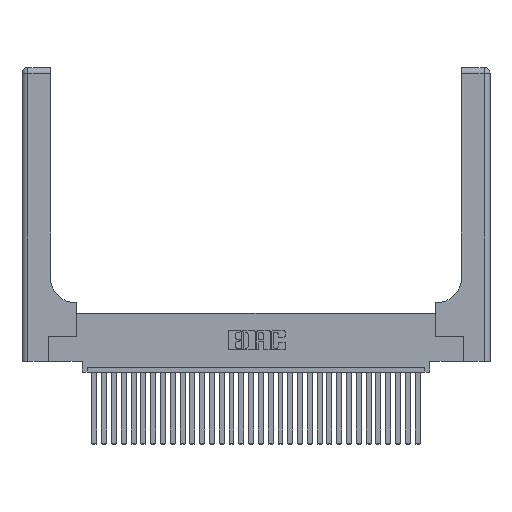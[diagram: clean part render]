
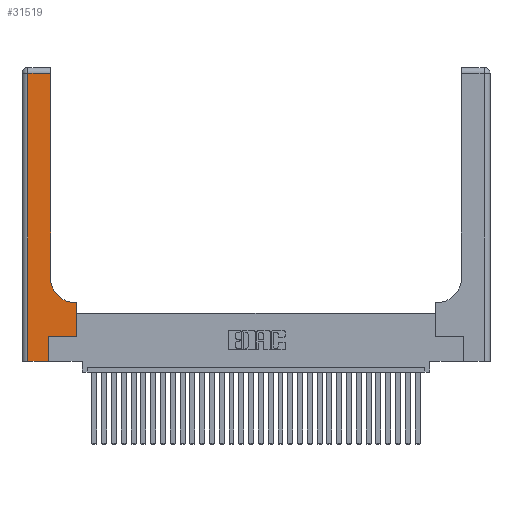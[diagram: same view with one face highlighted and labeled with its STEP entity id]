
A CAD part, top view. The second image highlights one B-rep face of the part: STEP entity #31519.
In plain terms, the highlighted planar face has unit normal (0, 0, 1).
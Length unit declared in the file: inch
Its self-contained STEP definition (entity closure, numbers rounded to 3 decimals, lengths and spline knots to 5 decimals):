
#230 = DIRECTION ( 'NONE',  ( -1., 0., 0. ) ) ;
#403 = CARTESIAN_POINT ( 'NONE',  ( 0.269, 0.25, 0.37 ) ) ;
#1255 = CARTESIAN_POINT ( 'NONE',  ( 0.06, 2.94, 0.37 ) ) ;
#1297 = VERTEX_POINT ( 'NONE', #24731 ) ;
#2402 = ORIENTED_EDGE ( 'NONE', *, *, #20501, .T. ) ;
#2521 = DIRECTION ( 'NONE',  ( 1., 0., 0. ) ) ;
#2644 = VERTEX_POINT ( 'NONE', #13445 ) ;
#3068 = CARTESIAN_POINT ( 'NONE',  ( 0.5585, 0.25, 0.37 ) ) ;
#3902 = ORIENTED_EDGE ( 'NONE', *, *, #19880, .T. ) ;
#4664 = CARTESIAN_POINT ( 'NONE',  ( 0.2915, 3., 0.37 ) ) ;
#4743 = ORIENTED_EDGE ( 'NONE', *, *, #15326, .T. ) ;
#5087 = CARTESIAN_POINT ( 'NONE',  ( 0.5415, 0.85, 0.37 ) ) ;
#5711 = DIRECTION ( 'NONE',  ( 0., 1., 0. ) ) ;
#5930 = FACE_OUTER_BOUND ( 'NONE', #12871, .T. ) ;
#6453 = ORIENTED_EDGE ( 'NONE', *, *, #16240, .T. ) ;
#6502 = CARTESIAN_POINT ( 'NONE',  ( 0., 3., 0.37 ) ) ;
#6890 = EDGE_CURVE ( 'NONE', #15821, #16080, #20571, .T. ) ;
#7287 = CARTESIAN_POINT ( 'NONE',  ( 0.269, 0., 0.37 ) ) ;
#8060 = EDGE_CURVE ( 'NONE', #1297, #13843, #15894, .T. ) ;
#8064 = EDGE_CURVE ( 'NONE', #21628, #1297, #30498, .T. ) ;
#8325 = DIRECTION ( 'NONE',  ( -1., 0., 0. ) ) ;
#8755 = CARTESIAN_POINT ( 'NONE',  ( 0.06, 0., 0.37 ) ) ;
#9092 = CARTESIAN_POINT ( 'NONE',  ( 0., 0., 0.37 ) ) ;
#9494 = LINE ( 'NONE', #11386, #15234 ) ;
#9733 = ORIENTED_EDGE ( 'NONE', *, *, #15636, .T. ) ;
#9889 = CARTESIAN_POINT ( 'NONE',  ( 0.06, 3., 0.37 ) ) ;
#10263 = CARTESIAN_POINT ( 'NONE',  ( 0.269, 0., 0.37 ) ) ;
#10297 = CARTESIAN_POINT ( 'NONE',  ( 0.2915, 2.94, 0.37 ) ) ;
#10461 = AXIS2_PLACEMENT_3D ( 'NONE', #6502, #17881, #8325 ) ;
#10474 = AXIS2_PLACEMENT_3D ( 'NONE', #5087, #22228, #2521 ) ;
#11088 = VERTEX_POINT ( 'NONE', #23471 ) ;
#11386 = CARTESIAN_POINT ( 'NONE',  ( 0., 2.94, 0.37 ) ) ;
#11417 = VERTEX_POINT ( 'NONE', #1255 ) ;
#11964 = VERTEX_POINT ( 'NONE', #10297 ) ;
#12871 = EDGE_LOOP ( 'NONE', ( #9733, #4743, #2402, #18147, #28691, #6453, #15661, #27315, #3902 ) ) ;
#13445 = CARTESIAN_POINT ( 'NONE',  ( 0.2915, 0.85, 0.37 ) ) ;
#13843 = VERTEX_POINT ( 'NONE', #17714 ) ;
#14063 = VECTOR ( 'NONE', #31431, 39.37008 ) ;
#14437 = DIRECTION ( 'NONE',  ( 0., 1., 0. ) ) ;
#14449 = VECTOR ( 'NONE', #14437, 39.37008 ) ;
#14633 = CIRCLE ( 'NONE', #10474, 0.25 ) ;
#15234 = VECTOR ( 'NONE', #230, 39.37008 ) ;
#15326 = EDGE_CURVE ( 'NONE', #11964, #11417, #9494, .T. ) ;
#15636 = EDGE_CURVE ( 'NONE', #2644, #11964, #25500, .T. ) ;
#15661 = ORIENTED_EDGE ( 'NONE', *, *, #8064, .T. ) ;
#15821 = VERTEX_POINT ( 'NONE', #8755 ) ;
#15894 = LINE ( 'NONE', #24783, #31292 ) ;
#16080 = VERTEX_POINT ( 'NONE', #7287 ) ;
#16240 = EDGE_CURVE ( 'NONE', #11088, #21628, #17098, .T. ) ;
#17098 = LINE ( 'NONE', #403, #27413 ) ;
#17714 = CARTESIAN_POINT ( 'NONE',  ( 0.5415, 0.6, 0.37 ) ) ;
#17881 = DIRECTION ( 'NONE',  ( 0., 0., -1. ) ) ;
#18147 = ORIENTED_EDGE ( 'NONE', *, *, #6890, .T. ) ;
#19449 = EDGE_CURVE ( 'NONE', #16080, #11088, #24570, .T. ) ;
#19880 = EDGE_CURVE ( 'NONE', #13843, #2644, #14633, .T. ) ;
#19956 = DIRECTION ( 'NONE',  ( 0., -1., 0. ) ) ;
#20021 = DIRECTION ( 'NONE',  ( 1., 0., 0. ) ) ;
#20225 = DIRECTION ( 'NONE',  ( 0., 1., 0. ) ) ;
#20501 = EDGE_CURVE ( 'NONE', #11417, #15821, #31067, .T. ) ;
#20571 = LINE ( 'NONE', #9092, #14063 ) ;
#21628 = VERTEX_POINT ( 'NONE', #25855 ) ;
#22228 = DIRECTION ( 'NONE',  ( 0., 0., -1. ) ) ;
#23471 = CARTESIAN_POINT ( 'NONE',  ( 0.269, 0.25, 0.37 ) ) ;
#24570 = LINE ( 'NONE', #10263, #31136 ) ;
#24731 = CARTESIAN_POINT ( 'NONE',  ( 0.5585, 0.6, 0.37 ) ) ;
#24783 = CARTESIAN_POINT ( 'NONE',  ( 0.2915, 0.6, 0.37 ) ) ;
#24999 = DIRECTION ( 'NONE',  ( -1., 0., 0. ) ) ;
#25500 = LINE ( 'NONE', #4664, #14449 ) ;
#25855 = CARTESIAN_POINT ( 'NONE',  ( 0.5585, 0.25, 0.37 ) ) ;
#27315 = ORIENTED_EDGE ( 'NONE', *, *, #8060, .T. ) ;
#27413 = VECTOR ( 'NONE', #20021, 39.37008 ) ;
#27951 = VECTOR ( 'NONE', #19956, 39.37008 ) ;
#28691 = ORIENTED_EDGE ( 'NONE', *, *, #19449, .T. ) ;
#30092 = PLANE ( 'NONE',  #10461 ) ;
#30498 = LINE ( 'NONE', #3068, #31659 ) ;
#31067 = LINE ( 'NONE', #9889, #27951 ) ;
#31136 = VECTOR ( 'NONE', #20225, 39.37008 ) ;
#31292 = VECTOR ( 'NONE', #24999, 39.37008 ) ;
#31431 = DIRECTION ( 'NONE',  ( 1., 0., 0. ) ) ;
#31519 = ADVANCED_FACE ( 'NONE', ( #5930 ), #30092, .F. ) ;
#31659 = VECTOR ( 'NONE', #5711, 39.37008 ) ;
